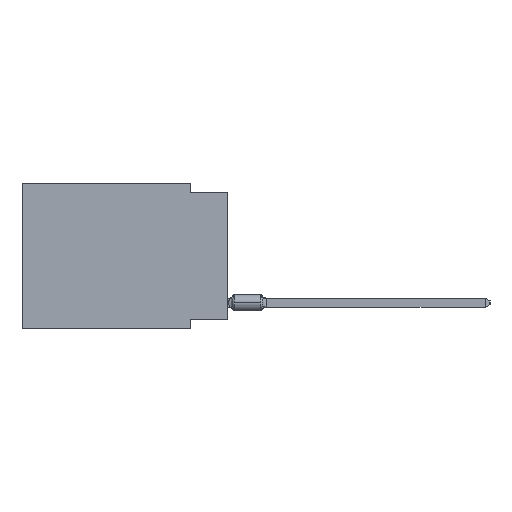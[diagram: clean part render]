
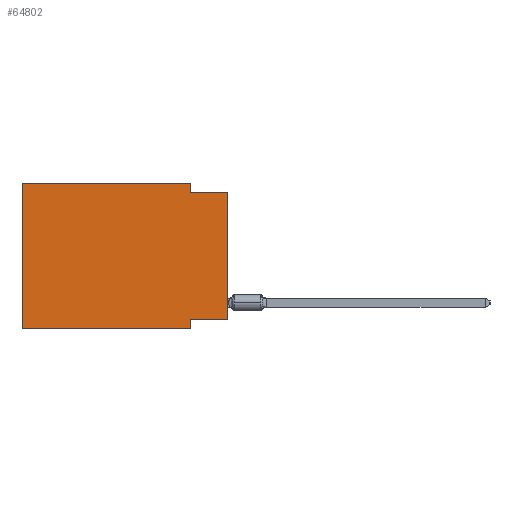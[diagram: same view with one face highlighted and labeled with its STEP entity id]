
A CAD part, left-side view. The second image highlights one B-rep face of the part: STEP entity #64802.
In plain terms, the highlighted planar face has unit normal (-1, 0, 0).
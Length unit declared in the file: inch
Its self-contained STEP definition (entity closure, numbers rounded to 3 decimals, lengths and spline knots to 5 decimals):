
#148 = CARTESIAN_POINT ( 'NONE',  ( 0., 0.1, 0. ) ) ;
#169 = ORIENTED_EDGE ( 'NONE', *, *, #55071, .F. ) ;
#680 = EDGE_LOOP ( 'NONE', ( #54208, #11830, #169, #56962, #45165, #47816, #51457, #10970 ) ) ;
#3057 = LINE ( 'NONE', #71353, #52983 ) ;
#5226 = VECTOR ( 'NONE', #39737, 39.37008 ) ;
#5950 = VECTOR ( 'NONE', #55746, 39.37008 ) ;
#6629 = CARTESIAN_POINT ( 'NONE',  ( 0., 0., -0.025 ) ) ;
#9000 = CARTESIAN_POINT ( 'NONE',  ( 0., 0., -0.025 ) ) ;
#9290 = DIRECTION ( 'NONE',  ( 0., 0., 1. ) ) ;
#9345 = DIRECTION ( 'NONE',  ( 0., 1., 0. ) ) ;
#10933 = LINE ( 'NONE', #16825, #5226 ) ;
#10970 = ORIENTED_EDGE ( 'NONE', *, *, #60794, .F. ) ;
#11830 = ORIENTED_EDGE ( 'NONE', *, *, #41720, .F. ) ;
#12619 = DIRECTION ( 'NONE',  ( 0., 0., -1. ) ) ;
#13947 = VECTOR ( 'NONE', #21123, 39.37008 ) ;
#15073 = VECTOR ( 'NONE', #39590, 39.37008 ) ;
#15427 = VERTEX_POINT ( 'NONE', #23273 ) ;
#15593 = LINE ( 'NONE', #27023, #13947 ) ;
#16825 = CARTESIAN_POINT ( 'NONE',  ( 0., 0.55, 0. ) ) ;
#17406 = DIRECTION ( 'NONE',  ( 1., 0., 0. ) ) ;
#17412 = CARTESIAN_POINT ( 'NONE',  ( 0., 0.55, -0.39 ) ) ;
#18349 = CARTESIAN_POINT ( 'NONE',  ( 0., 0.1, -0.39 ) ) ;
#18927 = VERTEX_POINT ( 'NONE', #55432 ) ;
#19263 = VECTOR ( 'NONE', #36850, 39.37008 ) ;
#20206 = LINE ( 'NONE', #70479, #19263 ) ;
#21123 = DIRECTION ( 'NONE',  ( 0., 0., -1. ) ) ;
#23273 = CARTESIAN_POINT ( 'NONE',  ( 0., 0.55, 0. ) ) ;
#24300 = VECTOR ( 'NONE', #29133, 39.37008 ) ;
#25088 = EDGE_CURVE ( 'NONE', #15427, #67588, #33182, .T. ) ;
#26909 = CARTESIAN_POINT ( 'NONE',  ( 0., 0.55, 0. ) ) ;
#27023 = CARTESIAN_POINT ( 'NONE',  ( 0., 0.1, -0.39 ) ) ;
#28112 = LINE ( 'NONE', #17412, #15073 ) ;
#29133 = DIRECTION ( 'NONE',  ( 0., -1., 0. ) ) ;
#29318 = VERTEX_POINT ( 'NONE', #31626 ) ;
#29583 = PLANE ( 'NONE',  #45232 ) ;
#31626 = CARTESIAN_POINT ( 'NONE',  ( 0., 0.1, -0.365 ) ) ;
#32217 = LINE ( 'NONE', #59608, #59026 ) ;
#33182 = LINE ( 'NONE', #26909, #5950 ) ;
#35220 = EDGE_CURVE ( 'NONE', #18927, #15427, #10933, .T. ) ;
#35833 = VERTEX_POINT ( 'NONE', #41945 ) ;
#36850 = DIRECTION ( 'NONE',  ( 0., 0., -1. ) ) ;
#39590 = DIRECTION ( 'NONE',  ( 0., -1., 0. ) ) ;
#39737 = DIRECTION ( 'NONE',  ( 0., 0., 1. ) ) ;
#41720 = EDGE_CURVE ( 'NONE', #35833, #46283, #52054, .T. ) ;
#41945 = CARTESIAN_POINT ( 'NONE',  ( 0., 0.1, -0.025 ) ) ;
#45165 = ORIENTED_EDGE ( 'NONE', *, *, #35220, .F. ) ;
#45232 = AXIS2_PLACEMENT_3D ( 'NONE', #68042, #17406, #12619 ) ;
#46283 = VERTEX_POINT ( 'NONE', #9000 ) ;
#47816 = ORIENTED_EDGE ( 'NONE', *, *, #70358, .T. ) ;
#50272 = EDGE_CURVE ( 'NONE', #54891, #46283, #3057, .T. ) ;
#51457 = ORIENTED_EDGE ( 'NONE', *, *, #70221, .F. ) ;
#52054 = LINE ( 'NONE', #6629, #24300 ) ;
#52983 = VECTOR ( 'NONE', #9290, 39.37008 ) ;
#53131 = CARTESIAN_POINT ( 'NONE',  ( 0., 0., -0.365 ) ) ;
#54208 = ORIENTED_EDGE ( 'NONE', *, *, #50272, .T. ) ;
#54891 = VERTEX_POINT ( 'NONE', #53131 ) ;
#55071 = EDGE_CURVE ( 'NONE', #67588, #35833, #20206, .T. ) ;
#55432 = CARTESIAN_POINT ( 'NONE',  ( 0., 0.55, -0.39 ) ) ;
#55746 = DIRECTION ( 'NONE',  ( 0., -1., 0. ) ) ;
#56962 = ORIENTED_EDGE ( 'NONE', *, *, #25088, .F. ) ;
#58167 = VERTEX_POINT ( 'NONE', #18349 ) ;
#59026 = VECTOR ( 'NONE', #9345, 39.37008 ) ;
#59608 = CARTESIAN_POINT ( 'NONE',  ( 0., 0., -0.365 ) ) ;
#60794 = EDGE_CURVE ( 'NONE', #54891, #29318, #32217, .T. ) ;
#63240 = FACE_OUTER_BOUND ( 'NONE', #680, .T. ) ;
#64802 = ADVANCED_FACE ( 'NONE', ( #63240 ), #29583, .F. ) ;
#67588 = VERTEX_POINT ( 'NONE', #148 ) ;
#68042 = CARTESIAN_POINT ( 'NONE',  ( 0., 0.55, 0. ) ) ;
#70221 = EDGE_CURVE ( 'NONE', #29318, #58167, #15593, .T. ) ;
#70358 = EDGE_CURVE ( 'NONE', #18927, #58167, #28112, .T. ) ;
#70479 = CARTESIAN_POINT ( 'NONE',  ( 0., 0.1, 0. ) ) ;
#71353 = CARTESIAN_POINT ( 'NONE',  ( 0., 0., 0. ) ) ;
